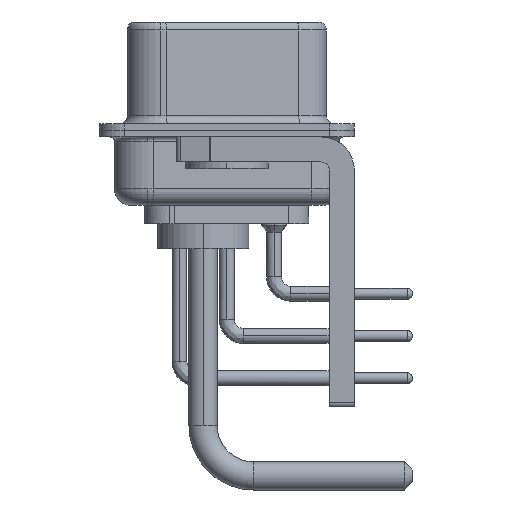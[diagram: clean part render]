
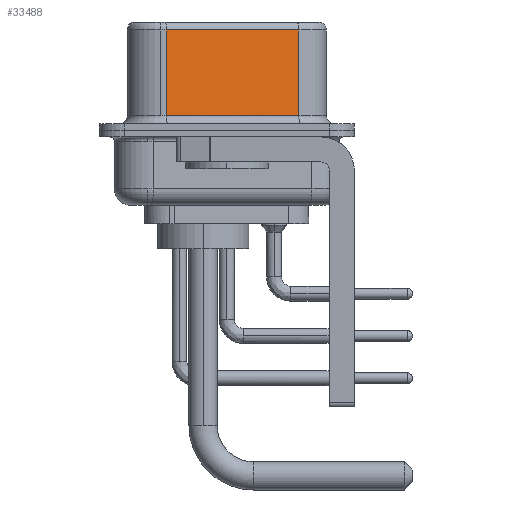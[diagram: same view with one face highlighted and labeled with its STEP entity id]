
A CAD part, left-side view. The second image highlights one B-rep face of the part: STEP entity #33488.
In plain terms, the highlighted planar face has unit normal (-0.985, -0.174, 0).
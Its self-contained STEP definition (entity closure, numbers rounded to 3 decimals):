
#496 = DIRECTION ( 'NONE',  ( -0.174, 0.985, 0. ) ) ;
#2072 = CARTESIAN_POINT ( 'NONE',  ( 3.73, 3.628, 6.02 ) ) ;
#2286 = DIRECTION ( 'NONE',  ( -0.174, 0.985, 0. ) ) ;
#4761 = CARTESIAN_POINT ( 'NONE',  ( 5.132, -4.322, 0.9 ) ) ;
#6081 = CARTESIAN_POINT ( 'NONE',  ( 5.132, -4.322, 6.02 ) ) ;
#6315 = VECTOR ( 'NONE', #31795, 1000. ) ;
#7279 = VECTOR ( 'NONE', #12922, 1000. ) ;
#7769 = CARTESIAN_POINT ( 'NONE',  ( 5.132, -4.322, 6.52 ) ) ;
#8154 = EDGE_CURVE ( 'NONE', #30260, #13865, #27392, .T. ) ;
#9895 = LINE ( 'NONE', #4761, #14782 ) ;
#10184 = ORIENTED_EDGE ( 'NONE', *, *, #24333, .T. ) ;
#12922 = DIRECTION ( 'NONE',  ( 0., 0., -1. ) ) ;
#13258 = CARTESIAN_POINT ( 'NONE',  ( 3.73, 3.628, 6.52 ) ) ;
#13865 = VERTEX_POINT ( 'NONE', #2072 ) ;
#14646 = ORIENTED_EDGE ( 'NONE', *, *, #8154, .T. ) ;
#14782 = VECTOR ( 'NONE', #28847, 1000. ) ;
#15551 = EDGE_CURVE ( 'NONE', #22796, #16932, #9895, .T. ) ;
#15685 = CARTESIAN_POINT ( 'NONE',  ( 5.132, -4.322, 6.52 ) ) ;
#16389 = ORIENTED_EDGE ( 'NONE', *, *, #32606, .F. ) ;
#16932 = VERTEX_POINT ( 'NONE', #17908 ) ;
#17908 = CARTESIAN_POINT ( 'NONE',  ( 5.132, -4.322, 0.9 ) ) ;
#18042 = LINE ( 'NONE', #13258, #7279 ) ;
#18953 = CARTESIAN_POINT ( 'NONE',  ( 3.73, 3.628, 0.9 ) ) ;
#20386 = FACE_OUTER_BOUND ( 'NONE', #27149, .T. ) ;
#21220 = DIRECTION ( 'NONE',  ( 0.985, 0.174, 0. ) ) ;
#22796 = VERTEX_POINT ( 'NONE', #18953 ) ;
#23141 = LINE ( 'NONE', #15685, #6315 ) ;
#24124 = ORIENTED_EDGE ( 'NONE', *, *, #15551, .T. ) ;
#24333 = EDGE_CURVE ( 'NONE', #13865, #22796, #18042, .T. ) ;
#24454 = AXIS2_PLACEMENT_3D ( 'NONE', #7769, #21220, #2286 ) ;
#25102 = CARTESIAN_POINT ( 'NONE',  ( 5.132, -4.322, 6.02 ) ) ;
#27149 = EDGE_LOOP ( 'NONE', ( #16389, #14646, #10184, #24124 ) ) ;
#27392 = LINE ( 'NONE', #25102, #32244 ) ;
#28847 = DIRECTION ( 'NONE',  ( 0.174, -0.985, 0. ) ) ;
#30260 = VERTEX_POINT ( 'NONE', #6081 ) ;
#31795 = DIRECTION ( 'NONE',  ( 0., 0., -1. ) ) ;
#32244 = VECTOR ( 'NONE', #496, 1000. ) ;
#32606 = EDGE_CURVE ( 'NONE', #30260, #16932, #23141, .T. ) ;
#33488 = ADVANCED_FACE ( 'NONE', ( #20386 ), #34666, .F. ) ;
#34666 = PLANE ( 'NONE',  #24454 ) ;
